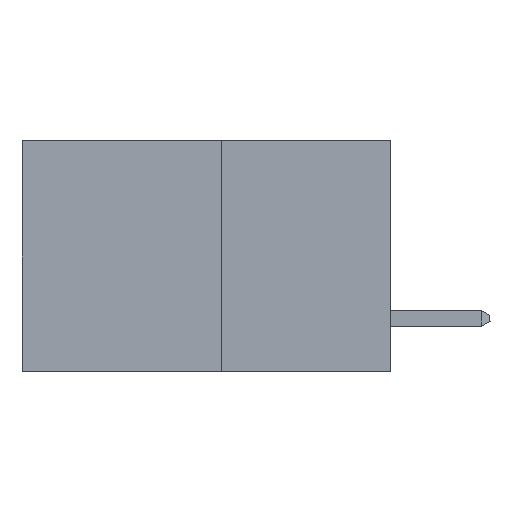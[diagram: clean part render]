
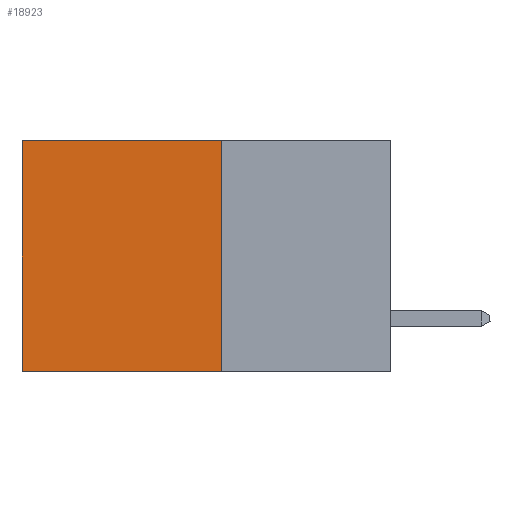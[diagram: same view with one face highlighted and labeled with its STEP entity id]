
A CAD part, left-side view. The second image highlights one B-rep face of the part: STEP entity #18923.
In plain terms, the highlighted planar face has unit normal (-1, 0, 0).
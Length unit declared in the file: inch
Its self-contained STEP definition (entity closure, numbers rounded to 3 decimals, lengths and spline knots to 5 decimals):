
#151 = VECTOR ( 'NONE', #12022, 39.37008 ) ;
#426 = CARTESIAN_POINT ( 'NONE',  ( 0.277, 0.27, -0.37 ) ) ;
#782 = ORIENTED_EDGE ( 'NONE', *, *, #2428, .F. ) ;
#1297 = AXIS2_PLACEMENT_3D ( 'NONE', #14666, #5770, #16111 ) ;
#1358 = VECTOR ( 'NONE', #4583, 39.37008 ) ;
#2428 = EDGE_CURVE ( 'NONE', #18495, #7262, #16102, .T. ) ;
#2499 = ORIENTED_EDGE ( 'NONE', *, *, #5040, .F. ) ;
#4296 = PLANE ( 'NONE',  #1297 ) ;
#4481 = CARTESIAN_POINT ( 'NONE',  ( 0.277, 0.59, -0.37 ) ) ;
#4583 = DIRECTION ( 'NONE',  ( 0., 0., -1. ) ) ;
#4756 = CARTESIAN_POINT ( 'NONE',  ( 0.277, 0.27, 0. ) ) ;
#5040 = EDGE_CURVE ( 'NONE', #7262, #8045, #9570, .T. ) ;
#5124 = VECTOR ( 'NONE', #16898, 39.37008 ) ;
#5460 = CARTESIAN_POINT ( 'NONE',  ( 0.277, 0.59, 0. ) ) ;
#5770 = DIRECTION ( 'NONE',  ( 1., 0., 0. ) ) ;
#5997 = CARTESIAN_POINT ( 'NONE',  ( 0.277, 0.59, -0.37 ) ) ;
#6795 = EDGE_CURVE ( 'NONE', #16438, #8045, #8607, .T. ) ;
#7262 = VERTEX_POINT ( 'NONE', #18744 ) ;
#8045 = VERTEX_POINT ( 'NONE', #5997 ) ;
#8607 = LINE ( 'NONE', #4481, #15956 ) ;
#8964 = DIRECTION ( 'NONE',  ( 0., 0., -1. ) ) ;
#9570 = LINE ( 'NONE', #13972, #5124 ) ;
#11927 = LINE ( 'NONE', #17840, #151 ) ;
#12022 = DIRECTION ( 'NONE',  ( 0., 1., 0. ) ) ;
#13972 = CARTESIAN_POINT ( 'NONE',  ( 0.277, 0.27, -0.37 ) ) ;
#14189 = ORIENTED_EDGE ( 'NONE', *, *, #6795, .T. ) ;
#14194 = ORIENTED_EDGE ( 'NONE', *, *, #17188, .T. ) ;
#14578 = EDGE_LOOP ( 'NONE', ( #14189, #2499, #782, #14194 ) ) ;
#14666 = CARTESIAN_POINT ( 'NONE',  ( 0.277, 0.27, -0.37 ) ) ;
#15956 = VECTOR ( 'NONE', #8964, 39.37008 ) ;
#16102 = LINE ( 'NONE', #426, #1358 ) ;
#16111 = DIRECTION ( 'NONE',  ( 0., 0., -1. ) ) ;
#16438 = VERTEX_POINT ( 'NONE', #5460 ) ;
#16898 = DIRECTION ( 'NONE',  ( 0., 1., 0. ) ) ;
#16915 = FACE_OUTER_BOUND ( 'NONE', #14578, .T. ) ;
#17188 = EDGE_CURVE ( 'NONE', #18495, #16438, #11927, .T. ) ;
#17840 = CARTESIAN_POINT ( 'NONE',  ( 0.277, 0.27, 0. ) ) ;
#18495 = VERTEX_POINT ( 'NONE', #4756 ) ;
#18744 = CARTESIAN_POINT ( 'NONE',  ( 0.277, 0.27, -0.37 ) ) ;
#18923 = ADVANCED_FACE ( 'NONE', ( #16915 ), #4296, .F. ) ;
